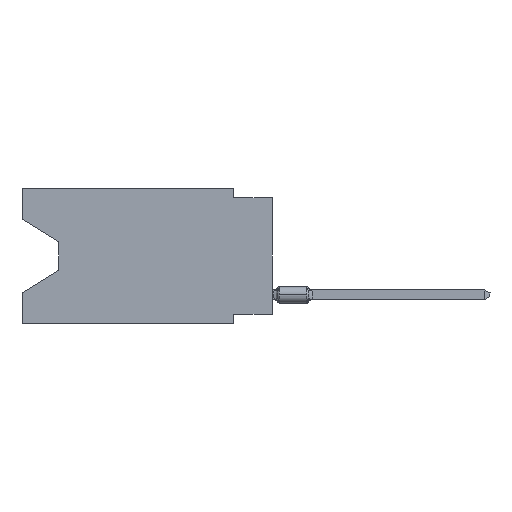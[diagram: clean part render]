
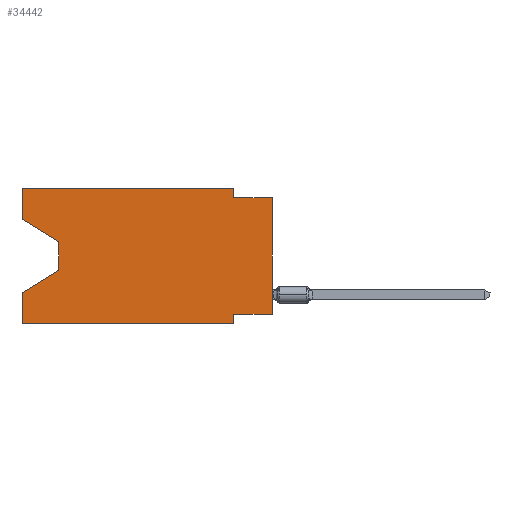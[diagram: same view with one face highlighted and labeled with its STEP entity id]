
A CAD part, left-side view. The second image highlights one B-rep face of the part: STEP entity #34442.
In plain terms, the highlighted planar face has unit normal (-1, 0, 0).
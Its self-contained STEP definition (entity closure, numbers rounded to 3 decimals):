
#914 = CARTESIAN_POINT ( 'NONE',  ( 0., 13.97, -3.505 ) ) ;
#1292 = VERTEX_POINT ( 'NONE', #25212 ) ;
#1830 = CARTESIAN_POINT ( 'NONE',  ( 0., 0., -0.635 ) ) ;
#2252 = VERTEX_POINT ( 'NONE', #44077 ) ;
#2330 = CARTESIAN_POINT ( 'NONE',  ( 0., 2.54, 0. ) ) ;
#2521 = CARTESIAN_POINT ( 'NONE',  ( 0., 16.383, 0. ) ) ;
#3820 = CARTESIAN_POINT ( 'NONE',  ( 0., 0., -8.255 ) ) ;
#4247 = VERTEX_POINT ( 'NONE', #23544 ) ;
#5007 = CARTESIAN_POINT ( 'NONE',  ( 0., 16.383, 0. ) ) ;
#5292 = PLANE ( 'NONE',  #40898 ) ;
#5839 = VECTOR ( 'NONE', #15801, 1000. ) ;
#6802 = LINE ( 'NONE', #36550, #13922 ) ;
#7320 = DIRECTION ( 'NONE',  ( 0., 0., -1. ) ) ;
#7505 = EDGE_CURVE ( 'NONE', #29827, #46968, #45498, .T. ) ;
#7905 = VECTOR ( 'NONE', #16774, 1000. ) ;
#8027 = CARTESIAN_POINT ( 'NONE',  ( 0., 2.54, -8.89 ) ) ;
#10075 = DIRECTION ( 'NONE',  ( 0., 0., 1. ) ) ;
#10402 = VECTOR ( 'NONE', #40144, 1000. ) ;
#10508 = EDGE_CURVE ( 'NONE', #45283, #1292, #38523, .T. ) ;
#10585 = DIRECTION ( 'NONE',  ( 0., -0.855, -0.519 ) ) ;
#11308 = ORIENTED_EDGE ( 'NONE', *, *, #37273, .T. ) ;
#13271 = VECTOR ( 'NONE', #16449, 1000. ) ;
#13588 = LINE ( 'NONE', #32342, #10402 ) ;
#13922 = VECTOR ( 'NONE', #40448, 1000. ) ;
#13991 = VECTOR ( 'NONE', #10585, 1000. ) ;
#14385 = CARTESIAN_POINT ( 'NONE',  ( 0., 16.383, -6.852 ) ) ;
#14492 = EDGE_CURVE ( 'NONE', #18151, #23499, #42058, .T. ) ;
#14813 = DIRECTION ( 'NONE',  ( 0., 0., 1. ) ) ;
#15089 = EDGE_CURVE ( 'NONE', #37128, #37357, #6802, .T. ) ;
#15321 = DIRECTION ( 'NONE',  ( 0., 0., -1. ) ) ;
#15801 = DIRECTION ( 'NONE',  ( 0., 0.855, -0.519 ) ) ;
#16129 = ORIENTED_EDGE ( 'NONE', *, *, #7505, .T. ) ;
#16174 = ORIENTED_EDGE ( 'NONE', *, *, #40608, .T. ) ;
#16209 = DIRECTION ( 'NONE',  ( 0., -1., 0. ) ) ;
#16449 = DIRECTION ( 'NONE',  ( 0., -1., 0. ) ) ;
#16497 = EDGE_CURVE ( 'NONE', #4247, #29827, #40336, .T. ) ;
#16676 = CARTESIAN_POINT ( 'NONE',  ( 0., 0., -0.635 ) ) ;
#16774 = DIRECTION ( 'NONE',  ( 0., 0., 1. ) ) ;
#16944 = CARTESIAN_POINT ( 'NONE',  ( 0., 13.97, -5.385 ) ) ;
#18151 = VERTEX_POINT ( 'NONE', #35721 ) ;
#18717 = VECTOR ( 'NONE', #42312, 1000. ) ;
#19044 = VECTOR ( 'NONE', #10075, 1000. ) ;
#19308 = CARTESIAN_POINT ( 'NONE',  ( 0., 13.97, -3.505 ) ) ;
#19904 = CARTESIAN_POINT ( 'NONE',  ( 0., 2.54, -8.89 ) ) ;
#19940 = VECTOR ( 'NONE', #15321, 1000. ) ;
#19988 = CARTESIAN_POINT ( 'NONE',  ( 0., 0., -8.255 ) ) ;
#20155 = CARTESIAN_POINT ( 'NONE',  ( 0., 16.383, 0. ) ) ;
#20450 = CARTESIAN_POINT ( 'NONE',  ( 0., 16.383, 0. ) ) ;
#20469 = EDGE_LOOP ( 'NONE', ( #29978, #16129, #16174, #46711, #40727, #35562, #25552, #11308, #32797, #21841, #42023, #23762 ) ) ;
#21007 = EDGE_CURVE ( 'NONE', #23499, #2252, #13588, .T. ) ;
#21841 = ORIENTED_EDGE ( 'NONE', *, *, #21007, .F. ) ;
#22648 = CARTESIAN_POINT ( 'NONE',  ( 0., 13.97, -5.385 ) ) ;
#23336 = CARTESIAN_POINT ( 'NONE',  ( 0., 16.383, -8.89 ) ) ;
#23499 = VERTEX_POINT ( 'NONE', #2330 ) ;
#23544 = CARTESIAN_POINT ( 'NONE',  ( 0., 16.383, -2.038 ) ) ;
#23762 = ORIENTED_EDGE ( 'NONE', *, *, #29885, .F. ) ;
#25212 = CARTESIAN_POINT ( 'NONE',  ( 0., 2.54, -8.255 ) ) ;
#25552 = ORIENTED_EDGE ( 'NONE', *, *, #10508, .F. ) ;
#28059 = DIRECTION ( 'NONE',  ( 0., 1., 0. ) ) ;
#29275 = EDGE_CURVE ( 'NONE', #2252, #33036, #43014, .T. ) ;
#29771 = DIRECTION ( 'NONE',  ( 1., 0., 0. ) ) ;
#29827 = VERTEX_POINT ( 'NONE', #19308 ) ;
#29885 = EDGE_CURVE ( 'NONE', #4247, #18151, #46049, .T. ) ;
#29978 = ORIENTED_EDGE ( 'NONE', *, *, #16497, .T. ) ;
#31527 = LINE ( 'NONE', #2521, #19044 ) ;
#32342 = CARTESIAN_POINT ( 'NONE',  ( 0., 2.54, 0. ) ) ;
#32797 = ORIENTED_EDGE ( 'NONE', *, *, #29275, .F. ) ;
#33036 = VERTEX_POINT ( 'NONE', #16676 ) ;
#33639 = FACE_OUTER_BOUND ( 'NONE', #20469, .T. ) ;
#33812 = LINE ( 'NONE', #38217, #34840 ) ;
#34292 = VERTEX_POINT ( 'NONE', #14385 ) ;
#34442 = ADVANCED_FACE ( 'NONE', ( #33639 ), #5292, .F. ) ;
#34840 = VECTOR ( 'NONE', #14813, 1000. ) ;
#35562 = ORIENTED_EDGE ( 'NONE', *, *, #35592, .F. ) ;
#35592 = EDGE_CURVE ( 'NONE', #1292, #37357, #41893, .T. ) ;
#35721 = CARTESIAN_POINT ( 'NONE',  ( 0., 16.383, 0. ) ) ;
#36470 = VECTOR ( 'NONE', #16209, 1000. ) ;
#36550 = CARTESIAN_POINT ( 'NONE',  ( 0., 16.383, -8.89 ) ) ;
#36689 = CARTESIAN_POINT ( 'NONE',  ( 0., 16.383, -2.038 ) ) ;
#37128 = VERTEX_POINT ( 'NONE', #23336 ) ;
#37273 = EDGE_CURVE ( 'NONE', #45283, #33036, #33812, .T. ) ;
#37357 = VERTEX_POINT ( 'NONE', #19904 ) ;
#37526 = LINE ( 'NONE', #22648, #5839 ) ;
#38217 = CARTESIAN_POINT ( 'NONE',  ( 0., 0., 0. ) ) ;
#38523 = LINE ( 'NONE', #19988, #38846 ) ;
#38846 = VECTOR ( 'NONE', #28059, 1000. ) ;
#39889 = EDGE_CURVE ( 'NONE', #37128, #34292, #31527, .T. ) ;
#40144 = DIRECTION ( 'NONE',  ( 0., 0., -1. ) ) ;
#40336 = LINE ( 'NONE', #36689, #13991 ) ;
#40448 = DIRECTION ( 'NONE',  ( 0., -1., 0. ) ) ;
#40608 = EDGE_CURVE ( 'NONE', #46968, #34292, #37526, .T. ) ;
#40727 = ORIENTED_EDGE ( 'NONE', *, *, #15089, .T. ) ;
#40898 = AXIS2_PLACEMENT_3D ( 'NONE', #20155, #29771, #7320 ) ;
#41893 = LINE ( 'NONE', #8027, #19940 ) ;
#42023 = ORIENTED_EDGE ( 'NONE', *, *, #14492, .F. ) ;
#42058 = LINE ( 'NONE', #5007, #36470 ) ;
#42312 = DIRECTION ( 'NONE',  ( 0., 0., -1. ) ) ;
#43014 = LINE ( 'NONE', #1830, #13271 ) ;
#44077 = CARTESIAN_POINT ( 'NONE',  ( 0., 2.54, -0.635 ) ) ;
#45283 = VERTEX_POINT ( 'NONE', #3820 ) ;
#45498 = LINE ( 'NONE', #914, #18717 ) ;
#46049 = LINE ( 'NONE', #20450, #7905 ) ;
#46711 = ORIENTED_EDGE ( 'NONE', *, *, #39889, .F. ) ;
#46968 = VERTEX_POINT ( 'NONE', #16944 ) ;
